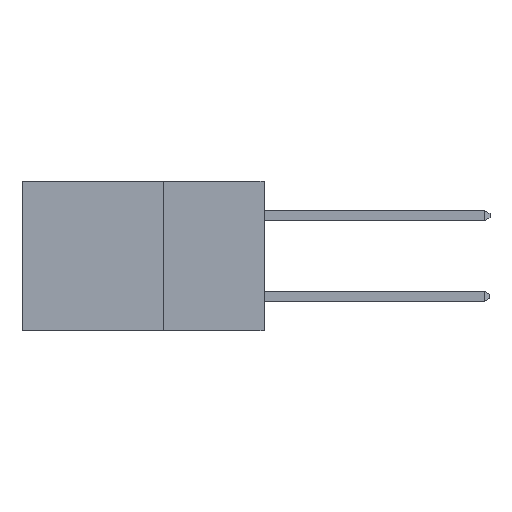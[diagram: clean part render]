
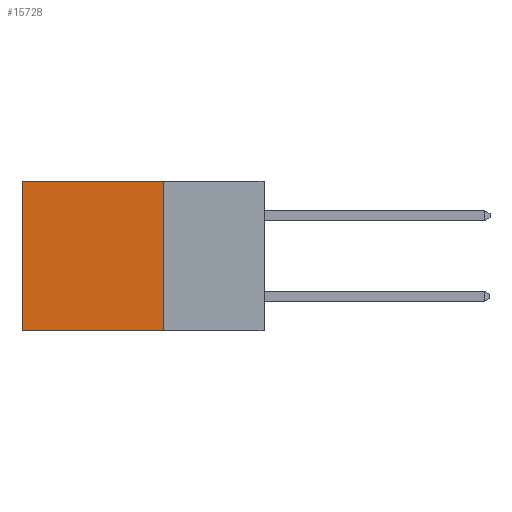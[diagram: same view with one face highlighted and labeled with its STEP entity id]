
A CAD part, left-side view. The second image highlights one B-rep face of the part: STEP entity #15728.
In plain terms, the highlighted planar face has unit normal (-1, 0, 0).
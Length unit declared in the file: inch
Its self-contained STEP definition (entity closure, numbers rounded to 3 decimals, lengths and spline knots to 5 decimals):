
#58 = AXIS2_PLACEMENT_3D ( 'NONE', #8807, #10377, #811 ) ;
#106 = ORIENTED_EDGE ( 'NONE', *, *, #4224, .F. ) ;
#764 = VERTEX_POINT ( 'NONE', #20248 ) ;
#811 = DIRECTION ( 'NONE',  ( 0., 0., -1. ) ) ;
#1379 = EDGE_CURVE ( 'NONE', #764, #10821, #11479, .T. ) ;
#2708 = CARTESIAN_POINT ( 'NONE',  ( 0.298, 0.6, 0. ) ) ;
#2792 = DIRECTION ( 'NONE',  ( 0., 1., 0. ) ) ;
#3754 = FACE_OUTER_BOUND ( 'NONE', #10717, .T. ) ;
#3809 = VERTEX_POINT ( 'NONE', #10713 ) ;
#3973 = ORIENTED_EDGE ( 'NONE', *, *, #7909, .T. ) ;
#4224 = EDGE_CURVE ( 'NONE', #3809, #10821, #9700, .T. ) ;
#4259 = LINE ( 'NONE', #18540, #16340 ) ;
#5551 = CARTESIAN_POINT ( 'NONE',  ( 0.298, 0.6, -0.37 ) ) ;
#6050 = VECTOR ( 'NONE', #12137, 39.37008 ) ;
#6506 = VERTEX_POINT ( 'NONE', #12278 ) ;
#7130 = PLANE ( 'NONE',  #58 ) ;
#7782 = VECTOR ( 'NONE', #13119, 39.37008 ) ;
#7909 = EDGE_CURVE ( 'NONE', #6506, #764, #4259, .T. ) ;
#8788 = ORIENTED_EDGE ( 'NONE', *, *, #15805, .F. ) ;
#8807 = CARTESIAN_POINT ( 'NONE',  ( 0.298, 0.25, 0. ) ) ;
#9700 = LINE ( 'NONE', #10909, #16981 ) ;
#10377 = DIRECTION ( 'NONE',  ( 1., 0., 0. ) ) ;
#10576 = CARTESIAN_POINT ( 'NONE',  ( 0.298, 0.25, 0. ) ) ;
#10579 = ORIENTED_EDGE ( 'NONE', *, *, #1379, .T. ) ;
#10713 = CARTESIAN_POINT ( 'NONE',  ( 0.298, 0.25, -0.37 ) ) ;
#10717 = EDGE_LOOP ( 'NONE', ( #10579, #106, #8788, #3973 ) ) ;
#10821 = VERTEX_POINT ( 'NONE', #5551 ) ;
#10909 = CARTESIAN_POINT ( 'NONE',  ( 0.298, 0.25, -0.37 ) ) ;
#11479 = LINE ( 'NONE', #2708, #7782 ) ;
#12137 = DIRECTION ( 'NONE',  ( 0., 0., -1. ) ) ;
#12278 = CARTESIAN_POINT ( 'NONE',  ( 0.298, 0.25, 0. ) ) ;
#12787 = DIRECTION ( 'NONE',  ( 0., 1., 0. ) ) ;
#13119 = DIRECTION ( 'NONE',  ( 0., 0., -1. ) ) ;
#15728 = ADVANCED_FACE ( 'NONE', ( #3754 ), #7130, .F. ) ;
#15805 = EDGE_CURVE ( 'NONE', #6506, #3809, #18020, .T. ) ;
#16340 = VECTOR ( 'NONE', #2792, 39.37008 ) ;
#16981 = VECTOR ( 'NONE', #12787, 39.37008 ) ;
#18020 = LINE ( 'NONE', #10576, #6050 ) ;
#18540 = CARTESIAN_POINT ( 'NONE',  ( 0.298, 0.25, 0. ) ) ;
#20248 = CARTESIAN_POINT ( 'NONE',  ( 0.298, 0.6, 0. ) ) ;
